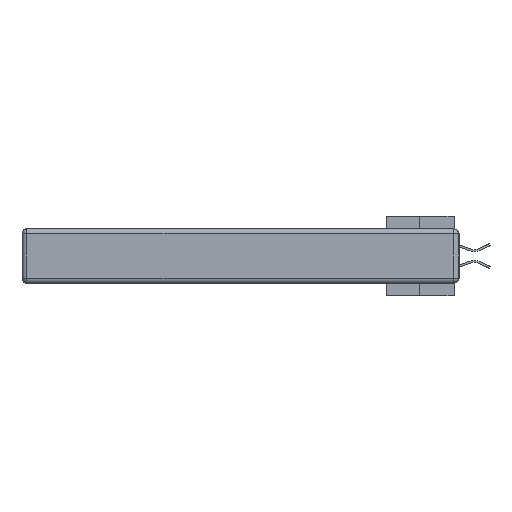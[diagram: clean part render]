
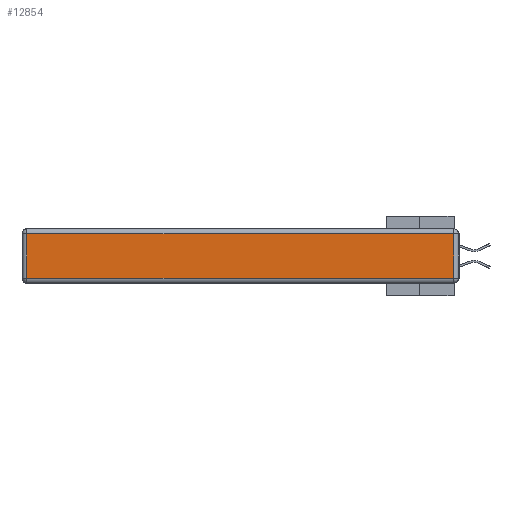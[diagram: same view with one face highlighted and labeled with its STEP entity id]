
A CAD part, left-side view. The second image highlights one B-rep face of the part: STEP entity #12854.
In plain terms, the highlighted planar face has unit normal (-1, 0, 0).
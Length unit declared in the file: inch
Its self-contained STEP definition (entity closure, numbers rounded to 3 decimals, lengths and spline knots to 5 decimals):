
#717 = CARTESIAN_POINT ( 'NONE',  ( 0., 0., -0.313 ) ) ;
#1954 = EDGE_CURVE ( 'NONE', #38066, #43935, #33601, .T. ) ;
#3127 = CARTESIAN_POINT ( 'NONE',  ( 0., 2.72, -0.03 ) ) ;
#6832 = CARTESIAN_POINT ( 'NONE',  ( 0., 0.03, -0.03 ) ) ;
#7248 = VECTOR ( 'NONE', #41430, 39.37008 ) ;
#7567 = LINE ( 'NONE', #717, #36203 ) ;
#7907 = VERTEX_POINT ( 'NONE', #34001 ) ;
#9379 = EDGE_CURVE ( 'NONE', #32211, #38066, #33504, .T. ) ;
#9388 = DIRECTION ( 'NONE',  ( 0., 0., 1. ) ) ;
#11715 = ORIENTED_EDGE ( 'NONE', *, *, #16010, .T. ) ;
#12854 = ADVANCED_FACE ( 'NONE', ( #40326 ), #26705, .T. ) ;
#16010 = EDGE_CURVE ( 'NONE', #7907, #32211, #7567, .T. ) ;
#18354 = EDGE_LOOP ( 'NONE', ( #11715, #38621, #37935, #35331 ) ) ;
#19220 = DIRECTION ( 'NONE',  ( 0., -1., 0. ) ) ;
#20880 = DIRECTION ( 'NONE',  ( 0., 1., 0. ) ) ;
#24492 = CARTESIAN_POINT ( 'NONE',  ( 0., 0.03, -0.313 ) ) ;
#25040 = CARTESIAN_POINT ( 'NONE',  ( 0., 0.03, -0.343 ) ) ;
#26705 = PLANE ( 'NONE',  #43965 ) ;
#32211 = VERTEX_POINT ( 'NONE', #24492 ) ;
#33444 = DIRECTION ( 'NONE',  ( -1., 0., 0. ) ) ;
#33504 = LINE ( 'NONE', #25040, #35729 ) ;
#33601 = LINE ( 'NONE', #34659, #38522 ) ;
#34001 = CARTESIAN_POINT ( 'NONE',  ( 0., 2.72, -0.313 ) ) ;
#34055 = CARTESIAN_POINT ( 'NONE',  ( 0., 0., -0.343 ) ) ;
#34514 = CARTESIAN_POINT ( 'NONE',  ( 0., 2.72, -0.343 ) ) ;
#34659 = CARTESIAN_POINT ( 'NONE',  ( 0., 2.75, -0.03 ) ) ;
#35331 = ORIENTED_EDGE ( 'NONE', *, *, #39065, .T. ) ;
#35729 = VECTOR ( 'NONE', #42621, 39.37008 ) ;
#36203 = VECTOR ( 'NONE', #19220, 39.37008 ) ;
#37935 = ORIENTED_EDGE ( 'NONE', *, *, #1954, .T. ) ;
#38066 = VERTEX_POINT ( 'NONE', #6832 ) ;
#38522 = VECTOR ( 'NONE', #20880, 39.37008 ) ;
#38621 = ORIENTED_EDGE ( 'NONE', *, *, #9379, .T. ) ;
#39065 = EDGE_CURVE ( 'NONE', #43935, #7907, #44155, .T. ) ;
#40326 = FACE_OUTER_BOUND ( 'NONE', #18354, .T. ) ;
#41430 = DIRECTION ( 'NONE',  ( 0., 0., -1. ) ) ;
#42621 = DIRECTION ( 'NONE',  ( 0., 0., 1. ) ) ;
#43935 = VERTEX_POINT ( 'NONE', #3127 ) ;
#43965 = AXIS2_PLACEMENT_3D ( 'NONE', #34055, #33444, #9388 ) ;
#44155 = LINE ( 'NONE', #34514, #7248 ) ;
